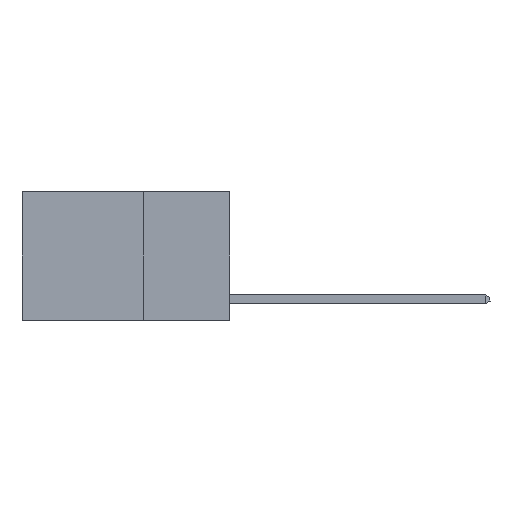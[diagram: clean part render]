
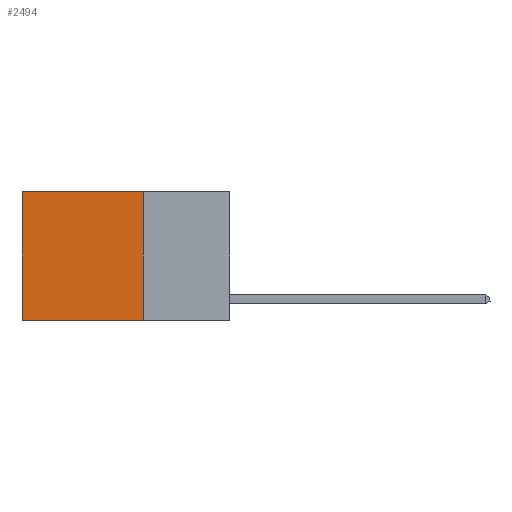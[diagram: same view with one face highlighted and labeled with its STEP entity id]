
A CAD part, left-side view. The second image highlights one B-rep face of the part: STEP entity #2494.
In plain terms, the highlighted planar face has unit normal (-1, 0, 0).
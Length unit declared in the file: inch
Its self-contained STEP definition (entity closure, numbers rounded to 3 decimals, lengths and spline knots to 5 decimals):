
#295 = ORIENTED_EDGE ( 'NONE', *, *, #13873, .T. ) ;
#301 = FACE_OUTER_BOUND ( 'NONE', #7687, .T. ) ;
#604 = CARTESIAN_POINT ( 'NONE',  ( 0.2625, 0.6, 0. ) ) ;
#1465 = LINE ( 'NONE', #15742, #1879 ) ;
#1556 = VERTEX_POINT ( 'NONE', #11396 ) ;
#1567 = VECTOR ( 'NONE', #7044, 39.37008 ) ;
#1879 = VECTOR ( 'NONE', #3913, 39.37008 ) ;
#1917 = PLANE ( 'NONE',  #10096 ) ;
#2494 = ADVANCED_FACE ( 'NONE', ( #301 ), #1917, .F. ) ;
#3139 = DIRECTION ( 'NONE',  ( 1., 0., 0. ) ) ;
#3357 = CARTESIAN_POINT ( 'NONE',  ( 0.2625, 0.25, 0. ) ) ;
#3835 = CARTESIAN_POINT ( 'NONE',  ( 0.2625, 0.25, -0.37 ) ) ;
#3913 = DIRECTION ( 'NONE',  ( 0., 1., 0. ) ) ;
#4299 = CARTESIAN_POINT ( 'NONE',  ( 0.2625, 0.25, 0. ) ) ;
#6817 = ORIENTED_EDGE ( 'NONE', *, *, #16746, .F. ) ;
#7044 = DIRECTION ( 'NONE',  ( 0., 1., 0. ) ) ;
#7322 = CARTESIAN_POINT ( 'NONE',  ( 0.2625, 0.6, -0.37 ) ) ;
#7687 = EDGE_LOOP ( 'NONE', ( #295, #12642, #6817, #10669 ) ) ;
#7875 = CARTESIAN_POINT ( 'NONE',  ( 0.2625, 0.6, 0. ) ) ;
#8176 = DIRECTION ( 'NONE',  ( 0., 0., -1. ) ) ;
#8306 = VERTEX_POINT ( 'NONE', #7322 ) ;
#8793 = VECTOR ( 'NONE', #16072, 39.37008 ) ;
#9103 = LINE ( 'NONE', #4299, #10978 ) ;
#10096 = AXIS2_PLACEMENT_3D ( 'NONE', #3357, #3139, #12384 ) ;
#10123 = EDGE_CURVE ( 'NONE', #14169, #8306, #14576, .T. ) ;
#10669 = ORIENTED_EDGE ( 'NONE', *, *, #16094, .T. ) ;
#10978 = VECTOR ( 'NONE', #8176, 39.37008 ) ;
#10992 = CARTESIAN_POINT ( 'NONE',  ( 0.2625, 0.25, -0.37 ) ) ;
#11396 = CARTESIAN_POINT ( 'NONE',  ( 0.2625, 0.25, 0. ) ) ;
#12384 = DIRECTION ( 'NONE',  ( 0., 0., -1. ) ) ;
#12642 = ORIENTED_EDGE ( 'NONE', *, *, #10123, .F. ) ;
#13873 = EDGE_CURVE ( 'NONE', #17082, #8306, #14562, .T. ) ;
#14169 = VERTEX_POINT ( 'NONE', #3835 ) ;
#14562 = LINE ( 'NONE', #604, #8793 ) ;
#14576 = LINE ( 'NONE', #10992, #1567 ) ;
#15742 = CARTESIAN_POINT ( 'NONE',  ( 0.2625, 0.25, 0. ) ) ;
#16072 = DIRECTION ( 'NONE',  ( 0., 0., -1. ) ) ;
#16094 = EDGE_CURVE ( 'NONE', #1556, #17082, #1465, .T. ) ;
#16746 = EDGE_CURVE ( 'NONE', #1556, #14169, #9103, .T. ) ;
#17082 = VERTEX_POINT ( 'NONE', #7875 ) ;
